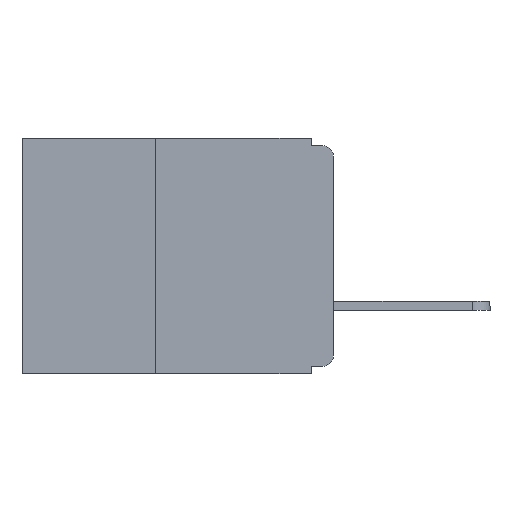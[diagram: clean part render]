
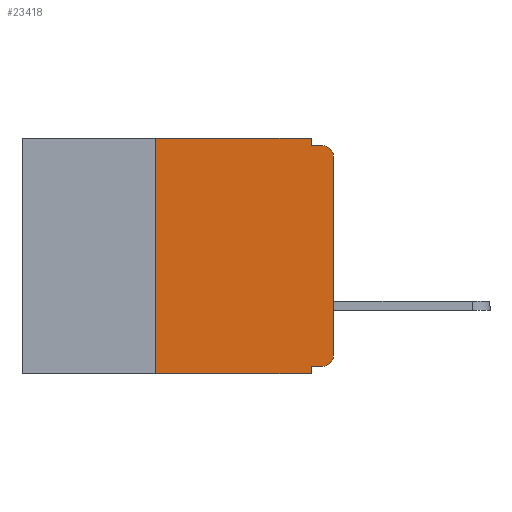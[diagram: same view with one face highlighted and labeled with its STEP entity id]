
A CAD part, left-side view. The second image highlights one B-rep face of the part: STEP entity #23418.
In plain terms, the highlighted planar face has unit normal (-1, 0, 0).
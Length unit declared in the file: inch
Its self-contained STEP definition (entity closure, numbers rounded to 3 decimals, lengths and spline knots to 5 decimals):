
#444 = DIRECTION ( 'NONE',  ( -1., 0., 0. ) ) ;
#578 = VERTEX_POINT ( 'NONE', #26327 ) ;
#769 = DIRECTION ( 'NONE',  ( 0., 0., 1. ) ) ;
#834 = CARTESIAN_POINT ( 'NONE',  ( 0., 0., -0.025 ) ) ;
#1008 = VERTEX_POINT ( 'NONE', #16713 ) ;
#1216 = AXIS2_PLACEMENT_3D ( 'NONE', #29813, #14155, #32453 ) ;
#1244 = CIRCLE ( 'NONE', #12750, 0.015 ) ;
#3190 = DIRECTION ( 'NONE',  ( 0., 0., -1. ) ) ;
#3370 = VERTEX_POINT ( 'NONE', #28183 ) ;
#4332 = EDGE_CURVE ( 'NONE', #7124, #1008, #27093, .T. ) ;
#4439 = CARTESIAN_POINT ( 'NONE',  ( 0., 0.031, -0.33 ) ) ;
#4602 = EDGE_CURVE ( 'NONE', #13015, #18288, #30358, .T. ) ;
#4709 = EDGE_CURVE ( 'NONE', #25278, #9930, #12350, .T. ) ;
#4846 = DIRECTION ( 'NONE',  ( 0., 0., 1. ) ) ;
#4904 = LINE ( 'NONE', #9666, #5764 ) ;
#5764 = VECTOR ( 'NONE', #25265, 39.37008 ) ;
#7124 = VERTEX_POINT ( 'NONE', #33508 ) ;
#7499 = EDGE_CURVE ( 'NONE', #7124, #13015, #11567, .T. ) ;
#8509 = VECTOR ( 'NONE', #30895, 39.37008 ) ;
#9533 = VECTOR ( 'NONE', #4846, 39.37008 ) ;
#9666 = CARTESIAN_POINT ( 'NONE',  ( 0., 0.437, -0.33 ) ) ;
#9930 = VERTEX_POINT ( 'NONE', #30207 ) ;
#9977 = ORIENTED_EDGE ( 'NONE', *, *, #7499, .T. ) ;
#10222 = CARTESIAN_POINT ( 'NONE',  ( 0., 0.437, 0. ) ) ;
#10609 = EDGE_LOOP ( 'NONE', ( #17376, #25558, #21093, #29727, #10965, #11393, #28578, #27208, #33015, #9977 ) ) ;
#10965 = ORIENTED_EDGE ( 'NONE', *, *, #4709, .F. ) ;
#11378 = AXIS2_PLACEMENT_3D ( 'NONE', #13624, #18969, #3190 ) ;
#11388 = EDGE_CURVE ( 'NONE', #9930, #20157, #15425, .T. ) ;
#11393 = ORIENTED_EDGE ( 'NONE', *, *, #13182, .F. ) ;
#11562 = VECTOR ( 'NONE', #11913, 39.37008 ) ;
#11567 = CIRCLE ( 'NONE', #1216, 0.015 ) ;
#11913 = DIRECTION ( 'NONE',  ( 0., 1., 0. ) ) ;
#12119 = LINE ( 'NONE', #4439, #18239 ) ;
#12350 = LINE ( 'NONE', #10222, #25405 ) ;
#12750 = AXIS2_PLACEMENT_3D ( 'NONE', #16375, #444, #18998 ) ;
#13015 = VERTEX_POINT ( 'NONE', #17395 ) ;
#13016 = CARTESIAN_POINT ( 'NONE',  ( 0., 0.25, 0. ) ) ;
#13085 = FACE_OUTER_BOUND ( 'NONE', #10609, .T. ) ;
#13182 = EDGE_CURVE ( 'NONE', #3370, #25278, #20776, .T. ) ;
#13624 = CARTESIAN_POINT ( 'NONE',  ( 0., 0.437, 0. ) ) ;
#14063 = EDGE_CURVE ( 'NONE', #1008, #23691, #12119, .T. ) ;
#14155 = DIRECTION ( 'NONE',  ( -1., 0., 0. ) ) ;
#14396 = EDGE_CURVE ( 'NONE', #18288, #578, #1244, .T. ) ;
#14971 = DIRECTION ( 'NONE',  ( 0., -1., 0. ) ) ;
#15120 = CARTESIAN_POINT ( 'NONE',  ( 0., 0.031, 0. ) ) ;
#15425 = LINE ( 'NONE', #15120, #8509 ) ;
#15955 = CARTESIAN_POINT ( 'NONE',  ( 0., 0.031, -0.01 ) ) ;
#16347 = PLANE ( 'NONE',  #11378 ) ;
#16375 = CARTESIAN_POINT ( 'NONE',  ( 0., 0.015, -0.025 ) ) ;
#16713 = CARTESIAN_POINT ( 'NONE',  ( 0., 0.031, -0.32 ) ) ;
#17376 = ORIENTED_EDGE ( 'NONE', *, *, #4602, .T. ) ;
#17395 = CARTESIAN_POINT ( 'NONE',  ( 0., 0., -0.305 ) ) ;
#18082 = DIRECTION ( 'NONE',  ( 0., -1., 0. ) ) ;
#18239 = VECTOR ( 'NONE', #22772, 39.37008 ) ;
#18288 = VERTEX_POINT ( 'NONE', #834 ) ;
#18969 = DIRECTION ( 'NONE',  ( 1., 0., 0. ) ) ;
#18998 = DIRECTION ( 'NONE',  ( 0., 0., -1. ) ) ;
#20157 = VERTEX_POINT ( 'NONE', #15955 ) ;
#20776 = LINE ( 'NONE', #29720, #33889 ) ;
#21093 = ORIENTED_EDGE ( 'NONE', *, *, #27433, .F. ) ;
#22772 = DIRECTION ( 'NONE',  ( 0., 0., -1. ) ) ;
#23418 = ADVANCED_FACE ( 'NONE', ( #13085 ), #16347, .F. ) ;
#23691 = VERTEX_POINT ( 'NONE', #30514 ) ;
#24464 = EDGE_CURVE ( 'NONE', #3370, #23691, #4904, .T. ) ;
#25265 = DIRECTION ( 'NONE',  ( 0., -1., 0. ) ) ;
#25278 = VERTEX_POINT ( 'NONE', #13016 ) ;
#25405 = VECTOR ( 'NONE', #18082, 39.37008 ) ;
#25558 = ORIENTED_EDGE ( 'NONE', *, *, #14396, .T. ) ;
#26327 = CARTESIAN_POINT ( 'NONE',  ( 0., 0.015, -0.01 ) ) ;
#27093 = LINE ( 'NONE', #30494, #11562 ) ;
#27208 = ORIENTED_EDGE ( 'NONE', *, *, #14063, .F. ) ;
#27433 = EDGE_CURVE ( 'NONE', #20157, #578, #34208, .T. ) ;
#28183 = CARTESIAN_POINT ( 'NONE',  ( 0., 0.25, -0.33 ) ) ;
#28578 = ORIENTED_EDGE ( 'NONE', *, *, #24464, .T. ) ;
#29147 = CARTESIAN_POINT ( 'NONE',  ( 0., 0., 0. ) ) ;
#29720 = CARTESIAN_POINT ( 'NONE',  ( 0., 0.25, -0.33 ) ) ;
#29727 = ORIENTED_EDGE ( 'NONE', *, *, #11388, .F. ) ;
#29813 = CARTESIAN_POINT ( 'NONE',  ( 0., 0.015, -0.305 ) ) ;
#30207 = CARTESIAN_POINT ( 'NONE',  ( 0., 0.031, 0. ) ) ;
#30358 = LINE ( 'NONE', #29147, #9533 ) ;
#30494 = CARTESIAN_POINT ( 'NONE',  ( 0., 0., -0.32 ) ) ;
#30514 = CARTESIAN_POINT ( 'NONE',  ( 0., 0.031, -0.33 ) ) ;
#30895 = DIRECTION ( 'NONE',  ( 0., 0., -1. ) ) ;
#32453 = DIRECTION ( 'NONE',  ( 0., 0., -1. ) ) ;
#33015 = ORIENTED_EDGE ( 'NONE', *, *, #4332, .F. ) ;
#33271 = CARTESIAN_POINT ( 'NONE',  ( 0., 0., -0.01 ) ) ;
#33377 = VECTOR ( 'NONE', #14971, 39.37008 ) ;
#33508 = CARTESIAN_POINT ( 'NONE',  ( 0., 0.015, -0.32 ) ) ;
#33889 = VECTOR ( 'NONE', #769, 39.37008 ) ;
#34208 = LINE ( 'NONE', #33271, #33377 ) ;
